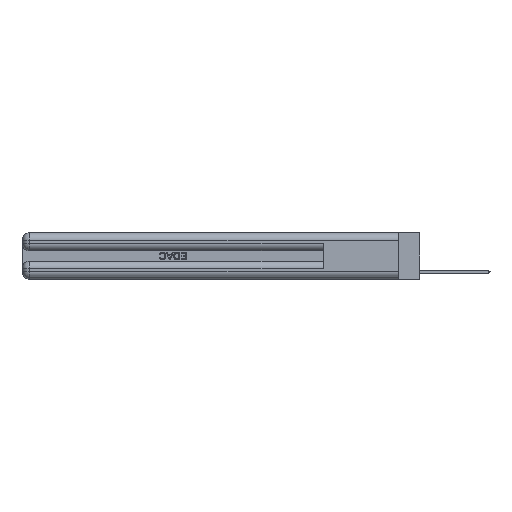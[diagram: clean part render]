
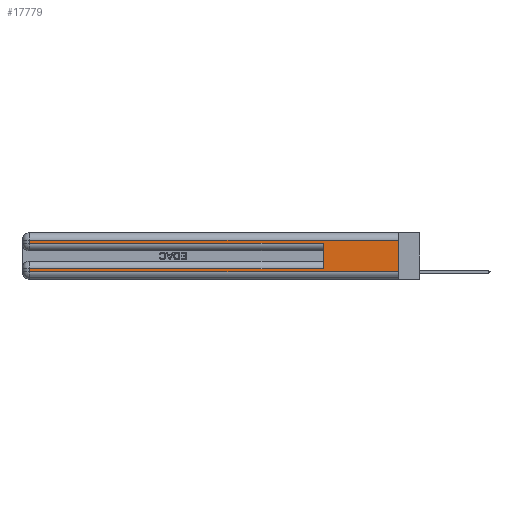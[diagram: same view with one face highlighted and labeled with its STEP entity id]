
A CAD part, left-side view. The second image highlights one B-rep face of the part: STEP entity #17779.
In plain terms, the highlighted planar face has unit normal (-1, 0, 0).
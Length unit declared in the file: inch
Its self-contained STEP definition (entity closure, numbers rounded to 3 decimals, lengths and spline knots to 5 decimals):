
#723 = PLANE ( 'NONE',  #10167 ) ;
#793 = VERTEX_POINT ( 'NONE', #18090 ) ;
#834 = DIRECTION ( 'NONE',  ( 0., 0., -1. ) ) ;
#1363 = VECTOR ( 'NONE', #5962, 39.37008 ) ;
#1386 = EDGE_CURVE ( 'NONE', #5108, #23774, #1954, .T. ) ;
#1431 = VECTOR ( 'NONE', #20035, 39.37008 ) ;
#1954 = LINE ( 'NONE', #20896, #21459 ) ;
#2452 = VERTEX_POINT ( 'NONE', #31004 ) ;
#4596 = FACE_OUTER_BOUND ( 'NONE', #14328, .T. ) ;
#5108 = VERTEX_POINT ( 'NONE', #11234 ) ;
#5315 = VECTOR ( 'NONE', #32176, 39.37008 ) ;
#5962 = DIRECTION ( 'NONE',  ( 0., 1., 0. ) ) ;
#6391 = CARTESIAN_POINT ( 'NONE',  ( 0., 0., 0.37 ) ) ;
#6401 = EDGE_CURVE ( 'NONE', #23484, #793, #21921, .T. ) ;
#6432 = DIRECTION ( 'NONE',  ( 0., -1., 0. ) ) ;
#7848 = VECTOR ( 'NONE', #25540, 39.37008 ) ;
#8275 = LINE ( 'NONE', #22190, #13312 ) ;
#8837 = DIRECTION ( 'NONE',  ( 1., 0., 0. ) ) ;
#9241 = VECTOR ( 'NONE', #33777, 39.37008 ) ;
#9701 = ORIENTED_EDGE ( 'NONE', *, *, #30707, .T. ) ;
#10167 = AXIS2_PLACEMENT_3D ( 'NONE', #6391, #8837, #834 ) ;
#10173 = EDGE_CURVE ( 'NONE', #16791, #793, #22115, .T. ) ;
#10242 = CARTESIAN_POINT ( 'NONE',  ( 0., 2.94, 0.085 ) ) ;
#10305 = EDGE_CURVE ( 'NONE', #23484, #23332, #13845, .T. ) ;
#10641 = CARTESIAN_POINT ( 'NONE',  ( 0., 0., 0.06 ) ) ;
#11234 = CARTESIAN_POINT ( 'NONE',  ( 0., 0., 0.31 ) ) ;
#12031 = DIRECTION ( 'NONE',  ( 0., -1., 0. ) ) ;
#13312 = VECTOR ( 'NONE', #6432, 39.37008 ) ;
#13845 = LINE ( 'NONE', #26055, #1363 ) ;
#14267 = LINE ( 'NONE', #25707, #9241 ) ;
#14328 = EDGE_LOOP ( 'NONE', ( #30839, #21399, #9701, #16574, #19163, #22619, #24936, #15656 ) ) ;
#14686 = VECTOR ( 'NONE', #12031, 39.37008 ) ;
#15656 = ORIENTED_EDGE ( 'NONE', *, *, #23059, .T. ) ;
#16574 = ORIENTED_EDGE ( 'NONE', *, *, #10173, .T. ) ;
#16791 = VERTEX_POINT ( 'NONE', #33409 ) ;
#17779 = ADVANCED_FACE ( 'NONE', ( #4596 ), #723, .F. ) ;
#17789 = DIRECTION ( 'NONE',  ( 0., 1., 0. ) ) ;
#18090 = CARTESIAN_POINT ( 'NONE',  ( 0., 0.6, 0.285 ) ) ;
#18452 = CARTESIAN_POINT ( 'NONE',  ( 0., 0.6, 0.145 ) ) ;
#18877 = LINE ( 'NONE', #32714, #1431 ) ;
#18961 = EDGE_CURVE ( 'NONE', #23332, #2452, #31830, .T. ) ;
#19163 = ORIENTED_EDGE ( 'NONE', *, *, #6401, .F. ) ;
#20035 = DIRECTION ( 'NONE',  ( 0., 0., -1. ) ) ;
#20896 = CARTESIAN_POINT ( 'NONE',  ( 0., 0., 0.31 ) ) ;
#21399 = ORIENTED_EDGE ( 'NONE', *, *, #1386, .T. ) ;
#21459 = VECTOR ( 'NONE', #17789, 39.37008 ) ;
#21921 = LINE ( 'NONE', #18452, #5315 ) ;
#22115 = LINE ( 'NONE', #27985, #14686 ) ;
#22190 = CARTESIAN_POINT ( 'NONE',  ( 0., 0., 0.06 ) ) ;
#22498 = CARTESIAN_POINT ( 'NONE',  ( 0., 2.94, 0.31 ) ) ;
#22619 = ORIENTED_EDGE ( 'NONE', *, *, #10305, .T. ) ;
#23059 = EDGE_CURVE ( 'NONE', #2452, #27362, #8275, .T. ) ;
#23332 = VERTEX_POINT ( 'NONE', #10242 ) ;
#23484 = VERTEX_POINT ( 'NONE', #31646 ) ;
#23774 = VERTEX_POINT ( 'NONE', #22498 ) ;
#24936 = ORIENTED_EDGE ( 'NONE', *, *, #18961, .T. ) ;
#25319 = CARTESIAN_POINT ( 'NONE',  ( 0., 2.94, 0.37 ) ) ;
#25540 = DIRECTION ( 'NONE',  ( 0., 0., -1. ) ) ;
#25707 = CARTESIAN_POINT ( 'NONE',  ( 0., 0., 0.37 ) ) ;
#26055 = CARTESIAN_POINT ( 'NONE',  ( 0., 0., 0.085 ) ) ;
#27362 = VERTEX_POINT ( 'NONE', #10641 ) ;
#27985 = CARTESIAN_POINT ( 'NONE',  ( 0., 0., 0.285 ) ) ;
#30707 = EDGE_CURVE ( 'NONE', #23774, #16791, #18877, .T. ) ;
#30839 = ORIENTED_EDGE ( 'NONE', *, *, #32067, .F. ) ;
#31004 = CARTESIAN_POINT ( 'NONE',  ( 0., 2.94, 0.06 ) ) ;
#31646 = CARTESIAN_POINT ( 'NONE',  ( 0., 0.6, 0.085 ) ) ;
#31830 = LINE ( 'NONE', #25319, #7848 ) ;
#32067 = EDGE_CURVE ( 'NONE', #5108, #27362, #14267, .T. ) ;
#32176 = DIRECTION ( 'NONE',  ( 0., 0., 1. ) ) ;
#32714 = CARTESIAN_POINT ( 'NONE',  ( 0., 2.94, 0.37 ) ) ;
#33409 = CARTESIAN_POINT ( 'NONE',  ( 0., 2.94, 0.285 ) ) ;
#33777 = DIRECTION ( 'NONE',  ( 0., 0., -1. ) ) ;
